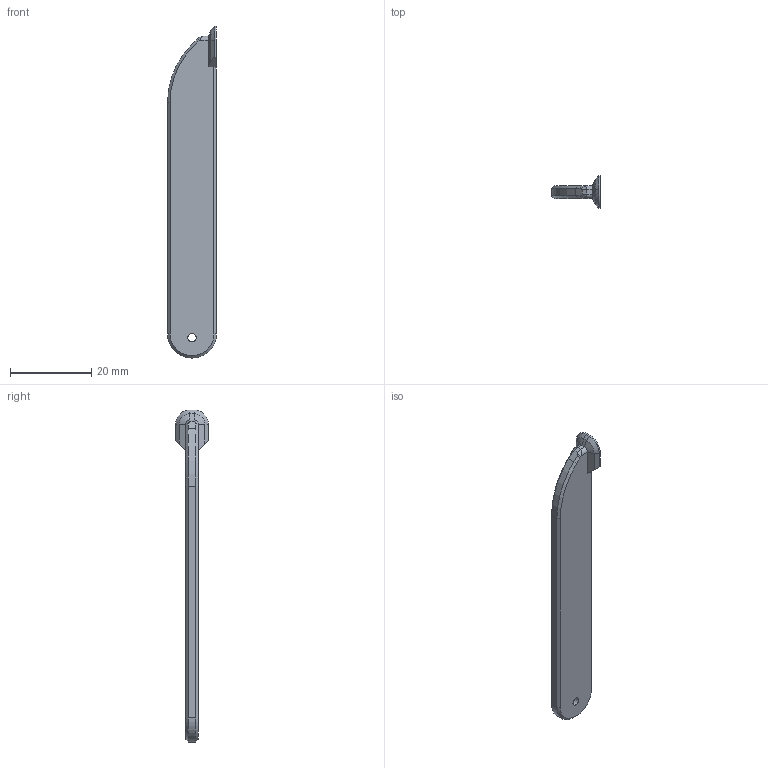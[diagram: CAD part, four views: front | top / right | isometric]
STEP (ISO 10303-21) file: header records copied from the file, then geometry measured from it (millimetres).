
FILE_DESCRIPTION(('FreeCAD Model'),'2;1');
FILE_NAME('Open CASCADE Shape Model','2022-10-05T16:42:12',('Author'),( ''),'Open CASCADE STEP processor 7.6','FreeCAD','Unknown');
FILE_SCHEMA(('AUTOMOTIVE_DESIGN { 1 0 10303 214 1 1 1 1 }'));
Length unit declared in the file: millimetre
Products named in the file (1): Fin001
Bounding box: 12 x 8 x 81.5 mm (x, y, z)
Volume: 2670.4 mm3; surface area: 2281 mm2
Topology: 1 solids, 1 shells, 49 faces, 115 edges, 68 vertices
Faces by surface type: plane 27, cone 10, cylinder 8, bspline 4
Full cylindrical faces by diameter (mm): 2 x1
Entity records: 2949 total; most frequent: CARTESIAN_POINT 701, DIRECTION 380, LINE 237, VECTOR 237, ORIENTED_EDGE 230, PCURVE 230, DEFINITIONAL_REPRESENTATION 230, EDGE_CURVE 115
